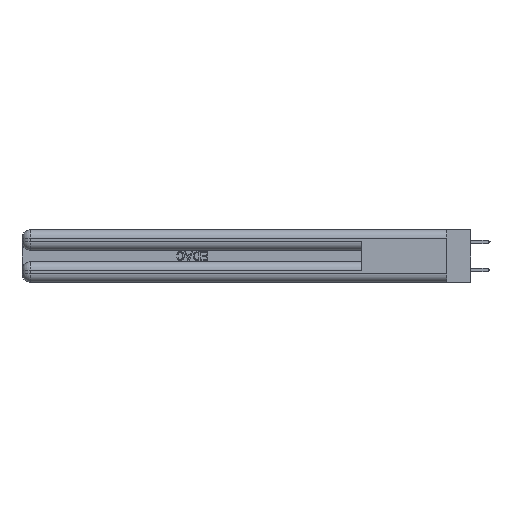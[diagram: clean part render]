
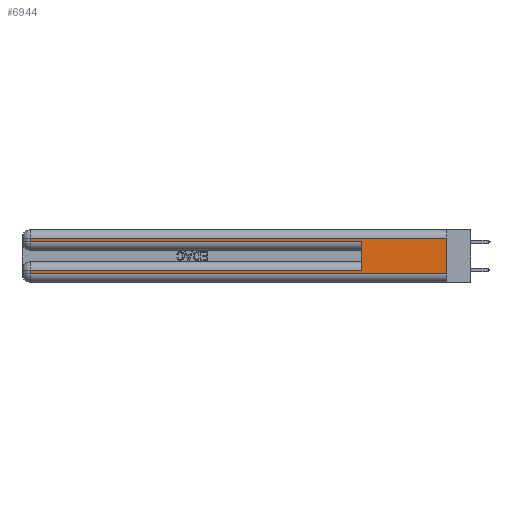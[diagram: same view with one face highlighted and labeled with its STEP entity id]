
A CAD part, left-side view. The second image highlights one B-rep face of the part: STEP entity #6944.
In plain terms, the highlighted planar face has unit normal (-1, 0, 0).
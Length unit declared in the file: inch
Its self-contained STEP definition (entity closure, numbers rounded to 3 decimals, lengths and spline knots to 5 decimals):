
#47 = CARTESIAN_POINT ( 'NONE',  ( 0., 2.94, 0.31 ) ) ;
#102 = VECTOR ( 'NONE', #4769, 39.37008 ) ;
#1109 = FACE_OUTER_BOUND ( 'NONE', #44401, .T. ) ;
#2033 = EDGE_CURVE ( 'NONE', #32724, #7515, #47541, .T. ) ;
#2593 = CARTESIAN_POINT ( 'NONE',  ( 0., 0., 0.37 ) ) ;
#2673 = VERTEX_POINT ( 'NONE', #16890 ) ;
#3478 = CARTESIAN_POINT ( 'NONE',  ( 0., 0., 0.06 ) ) ;
#3487 = CARTESIAN_POINT ( 'NONE',  ( 0., 0., 0.37 ) ) ;
#4162 = VECTOR ( 'NONE', #29282, 39.37008 ) ;
#4769 = DIRECTION ( 'NONE',  ( 0., 0., -1. ) ) ;
#5318 = ORIENTED_EDGE ( 'NONE', *, *, #34193, .T. ) ;
#6944 = ADVANCED_FACE ( 'NONE', ( #1109 ), #7398, .F. ) ;
#7217 = ORIENTED_EDGE ( 'NONE', *, *, #2033, .T. ) ;
#7383 = VECTOR ( 'NONE', #10147, 39.37008 ) ;
#7398 = PLANE ( 'NONE',  #11526 ) ;
#7502 = VERTEX_POINT ( 'NONE', #18458 ) ;
#7515 = VERTEX_POINT ( 'NONE', #41167 ) ;
#8176 = ORIENTED_EDGE ( 'NONE', *, *, #30346, .T. ) ;
#8271 = CARTESIAN_POINT ( 'NONE',  ( 0., 0., 0.31 ) ) ;
#9665 = EDGE_CURVE ( 'NONE', #39108, #2673, #46614, .T. ) ;
#10147 = DIRECTION ( 'NONE',  ( 0., 1., 0. ) ) ;
#11044 = DIRECTION ( 'NONE',  ( 0., 0., -1. ) ) ;
#11373 = CARTESIAN_POINT ( 'NONE',  ( 0., 2.94, 0.085 ) ) ;
#11526 = AXIS2_PLACEMENT_3D ( 'NONE', #3487, #34444, #41849 ) ;
#13612 = DIRECTION ( 'NONE',  ( 0., -1., 0. ) ) ;
#14218 = ORIENTED_EDGE ( 'NONE', *, *, #44193, .F. ) ;
#16890 = CARTESIAN_POINT ( 'NONE',  ( 0., 2.94, 0.285 ) ) ;
#16899 = CARTESIAN_POINT ( 'NONE',  ( 0., 0.6, 0.285 ) ) ;
#16958 = EDGE_CURVE ( 'NONE', #43119, #39108, #38771, .T. ) ;
#18458 = CARTESIAN_POINT ( 'NONE',  ( 0., 0.6, 0.085 ) ) ;
#20517 = CARTESIAN_POINT ( 'NONE',  ( 0., 0.6, 0.145 ) ) ;
#20674 = LINE ( 'NONE', #20517, #24917 ) ;
#21110 = VERTEX_POINT ( 'NONE', #3478 ) ;
#21144 = DIRECTION ( 'NONE',  ( 0., 1., 0. ) ) ;
#21320 = LINE ( 'NONE', #36765, #43072 ) ;
#22124 = EDGE_CURVE ( 'NONE', #7502, #32724, #38231, .T. ) ;
#24917 = VECTOR ( 'NONE', #47849, 39.37008 ) ;
#29282 = DIRECTION ( 'NONE',  ( 0., -1., 0. ) ) ;
#30346 = EDGE_CURVE ( 'NONE', #7515, #21110, #32037, .T. ) ;
#32037 = LINE ( 'NONE', #37549, #4162 ) ;
#32724 = VERTEX_POINT ( 'NONE', #11373 ) ;
#33623 = CARTESIAN_POINT ( 'NONE',  ( 0., 0., 0.085 ) ) ;
#33930 = VECTOR ( 'NONE', #21144, 39.37008 ) ;
#34193 = EDGE_CURVE ( 'NONE', #2673, #39923, #21320, .T. ) ;
#34444 = DIRECTION ( 'NONE',  ( 1., 0., 0. ) ) ;
#34487 = LINE ( 'NONE', #2593, #43519 ) ;
#36765 = CARTESIAN_POINT ( 'NONE',  ( 0., 0., 0.285 ) ) ;
#37549 = CARTESIAN_POINT ( 'NONE',  ( 0., 0., 0.06 ) ) ;
#38231 = LINE ( 'NONE', #33623, #7383 ) ;
#38771 = LINE ( 'NONE', #47961, #33930 ) ;
#39108 = VERTEX_POINT ( 'NONE', #47 ) ;
#39884 = DIRECTION ( 'NONE',  ( 0., 0., -1. ) ) ;
#39923 = VERTEX_POINT ( 'NONE', #16899 ) ;
#40906 = VECTOR ( 'NONE', #39884, 39.37008 ) ;
#41167 = CARTESIAN_POINT ( 'NONE',  ( 0., 2.94, 0.06 ) ) ;
#41849 = DIRECTION ( 'NONE',  ( 0., 0., -1. ) ) ;
#42133 = EDGE_CURVE ( 'NONE', #7502, #39923, #20674, .T. ) ;
#42799 = ORIENTED_EDGE ( 'NONE', *, *, #22124, .T. ) ;
#42964 = CARTESIAN_POINT ( 'NONE',  ( 0., 2.94, 0.37 ) ) ;
#43072 = VECTOR ( 'NONE', #13612, 39.37008 ) ;
#43119 = VERTEX_POINT ( 'NONE', #8271 ) ;
#43519 = VECTOR ( 'NONE', #11044, 39.37008 ) ;
#43540 = ORIENTED_EDGE ( 'NONE', *, *, #42133, .F. ) ;
#43741 = CARTESIAN_POINT ( 'NONE',  ( 0., 2.94, 0.37 ) ) ;
#44193 = EDGE_CURVE ( 'NONE', #43119, #21110, #34487, .T. ) ;
#44401 = EDGE_LOOP ( 'NONE', ( #14218, #47423, #48755, #5318, #43540, #42799, #7217, #8176 ) ) ;
#46614 = LINE ( 'NONE', #42964, #102 ) ;
#47423 = ORIENTED_EDGE ( 'NONE', *, *, #16958, .T. ) ;
#47541 = LINE ( 'NONE', #43741, #40906 ) ;
#47849 = DIRECTION ( 'NONE',  ( 0., 0., 1. ) ) ;
#47961 = CARTESIAN_POINT ( 'NONE',  ( 0., 0., 0.31 ) ) ;
#48755 = ORIENTED_EDGE ( 'NONE', *, *, #9665, .T. ) ;
